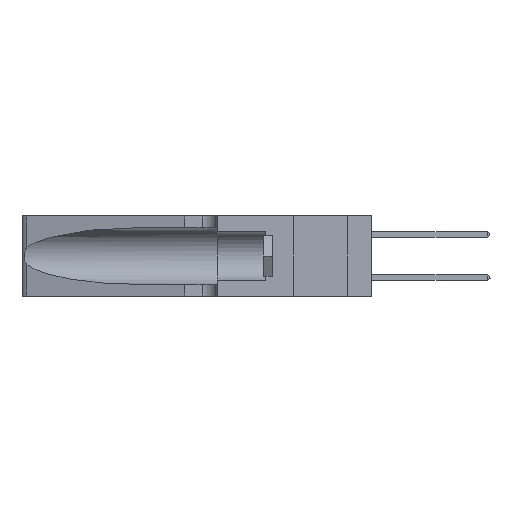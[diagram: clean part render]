
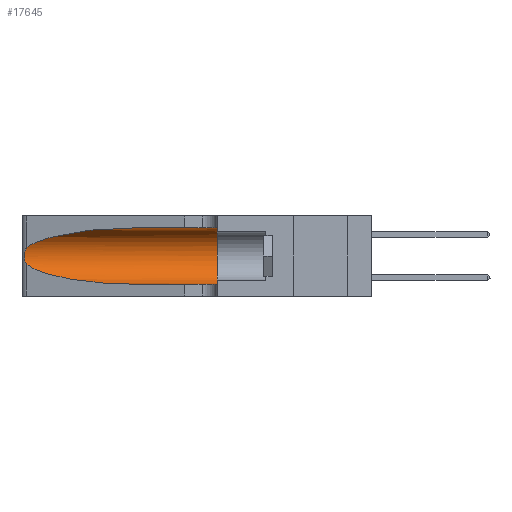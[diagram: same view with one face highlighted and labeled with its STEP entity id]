
A CAD part, left-side view. The second image highlights one B-rep face of the part: STEP entity #17645.
In plain terms, the highlighted cylindrical face has radius 3.308 mm (diameter 6.617 mm), a partial arc.
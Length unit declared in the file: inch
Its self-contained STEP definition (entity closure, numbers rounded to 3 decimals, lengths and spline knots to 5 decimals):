
#601 = CARTESIAN_POINT ( 'NONE',  ( 0.25789, 1.23486, 0.15765 ) ) ;
#664 = EDGE_CURVE ( 'NONE', #21509, #12738, #28038, .T. ) ;
#1256 = VECTOR ( 'NONE', #7456, 39.37008 ) ;
#2306 = CARTESIAN_POINT ( 'NONE',  ( 0.25487, 1.22718, 0.22369 ) ) ;
#3227 = CARTESIAN_POINT ( 'NONE',  ( 0.1305, 0.72297, 0.31525 ) ) ;
#3521 = CARTESIAN_POINT ( 'NONE',  ( 0.1305, 1.61858, 0.05475 ) ) ;
#4087 = FACE_OUTER_BOUND ( 'NONE', #15825, .T. ) ;
#4852 = CARTESIAN_POINT ( 'NONE',  ( 0.1305, 1.61858, 0.31525 ) ) ;
#5304 = AXIS2_PLACEMENT_3D ( 'NONE', #11814, #27728, #27369 ) ;
#5886 = ORIENTED_EDGE ( 'NONE', *, *, #25168, .T. ) ;
#6325 = DIRECTION ( 'NONE',  ( 0., -1., 0. ) ) ;
#6662 = CARTESIAN_POINT ( 'NONE',  ( 0.25487, 1.22718, 0.14631 ) ) ;
#6696 =( BOUNDED_CURVE ( )  B_SPLINE_CURVE ( 3, ( #14615, #17452, #19934, #24827 ),
 .UNSPECIFIED., .F., .F. ) 
 B_SPLINE_CURVE_WITH_KNOTS ( ( 4, 4 ),
 ( 1.5708, 2.84003 ),
 .UNSPECIFIED. ) 
 CURVE ( )  GEOMETRIC_REPRESENTATION_ITEM ( )  RATIONAL_B_SPLINE_CURVE ( ( 1., 0.87, 0.87, 1. ) ) 
 REPRESENTATION_ITEM ( '' )  );
#7092 = CARTESIAN_POINT ( 'NONE',  ( 0.1305, 0.72297, 0.05475 ) ) ;
#7456 = DIRECTION ( 'NONE',  ( 0., -1., 0. ) ) ;
#7496 = CARTESIAN_POINT ( 'NONE',  ( 0.26018, 1.23835, 0.19895 ) ) ;
#8985 = CARTESIAN_POINT ( 'NONE',  ( 0.25487, 1.22718, 0.14631 ) ) ;
#9748 = CARTESIAN_POINT ( 'NONE',  ( 0.25555, 1.22994, 0.2215 ) ) ;
#10372 = ORIENTED_EDGE ( 'NONE', *, *, #21077, .T. ) ;
#10446 = EDGE_CURVE ( 'NONE', #28811, #21509, #25939, .T. ) ;
#10840 = VERTEX_POINT ( 'NONE', #25632 ) ;
#11349 = CARTESIAN_POINT ( 'NONE',  ( 0.1305, 0.72297, 0.05475 ) ) ;
#11554 = LINE ( 'NONE', #3521, #21632 ) ;
#11681 = DIRECTION ( 'NONE',  ( 0., -1., 0. ) ) ;
#11778 = CIRCLE ( 'NONE', #5304, 0.13025 ) ;
#11814 = CARTESIAN_POINT ( 'NONE',  ( 0.1305, 0.35, 0.185 ) ) ;
#12738 = VERTEX_POINT ( 'NONE', #7092 ) ;
#14615 = CARTESIAN_POINT ( 'NONE',  ( 0.1305, 0.72297, 0.31525 ) ) ;
#14930 = CARTESIAN_POINT ( 'NONE',  ( 0.26017, 1.23833, 0.17102 ) ) ;
#14951 = ORIENTED_EDGE ( 'NONE', *, *, #29182, .F. ) ;
#15768 = CYLINDRICAL_SURFACE ( 'NONE', #17881, 0.13025 ) ;
#15825 = EDGE_LOOP ( 'NONE', ( #5886, #29830, #28706, #10372, #16165, #14951 ) ) ;
#16165 = ORIENTED_EDGE ( 'NONE', *, *, #17404, .F. ) ;
#16203 = VERTEX_POINT ( 'NONE', #17660 ) ;
#17404 = EDGE_CURVE ( 'NONE', #16203, #10840, #11778, .T. ) ;
#17430 = LINE ( 'NONE', #4852, #1256 ) ;
#17452 = CARTESIAN_POINT ( 'NONE',  ( 0.18966, 0.96281, 0.31525 ) ) ;
#17645 = ADVANCED_FACE ( 'NONE', ( #4087 ), #15768, .F. ) ;
#17660 = CARTESIAN_POINT ( 'NONE',  ( 0.1305, 0.35, 0.31525 ) ) ;
#17865 = CARTESIAN_POINT ( 'NONE',  ( 0.25787, 1.23484, 0.2124 ) ) ;
#17881 = AXIS2_PLACEMENT_3D ( 'NONE', #23623, #11681, #32170 ) ;
#17935 = CARTESIAN_POINT ( 'NONE',  ( 0.25856, 1.23593, 0.16098 ) ) ;
#19042 = CARTESIAN_POINT ( 'NONE',  ( 0.25487, 1.22718, 0.22369 ) ) ;
#19075 = VERTEX_POINT ( 'NONE', #3227 ) ;
#19934 = CARTESIAN_POINT ( 'NONE',  ( 0.2373, 1.15595, 0.28018 ) ) ;
#21077 = EDGE_CURVE ( 'NONE', #12738, #10840, #11554, .T. ) ;
#21247 = CARTESIAN_POINT ( 'NONE',  ( 0.25639, 1.23186, 0.15144 ) ) ;
#21509 = VERTEX_POINT ( 'NONE', #6662 ) ;
#21632 = VECTOR ( 'NONE', #6325, 39.37008 ) ;
#22580 = CARTESIAN_POINT ( 'NONE',  ( 0.26075, 1.23896, 0.19203 ) ) ;
#22929 = CARTESIAN_POINT ( 'NONE',  ( 0.25854, 1.2359, 0.20912 ) ) ;
#23623 = CARTESIAN_POINT ( 'NONE',  ( 0.1305, 1.61858, 0.185 ) ) ;
#24827 = CARTESIAN_POINT ( 'NONE',  ( 0.25487, 1.22718, 0.22369 ) ) ;
#25168 = EDGE_CURVE ( 'NONE', #19075, #28811, #6696, .T. ) ;
#25632 = CARTESIAN_POINT ( 'NONE',  ( 0.1305, 0.35, 0.05475 ) ) ;
#25939 = B_SPLINE_CURVE_WITH_KNOTS ( 'NONE', 3,
 ( #2306, #9748, #32837, #17865, #22929, #7496, #22580, #30347, #14930, #17935, #601, #21247, #29220, #29109 ),
 .UNSPECIFIED., .F., .F.,
 ( 4, 2, 2, 2, 2, 2, 4 ),
 ( 0., 0.00027, 0.00053, 0.00107, 0.0016, 0.00187, 0.00214 ),
 .UNSPECIFIED. ) ;
#27121 = CARTESIAN_POINT ( 'NONE',  ( 0.2373, 1.15595, 0.08982 ) ) ;
#27369 = DIRECTION ( 'NONE',  ( 0., 0., 1. ) ) ;
#27728 = DIRECTION ( 'NONE',  ( 0., 1., 0. ) ) ;
#28038 =( BOUNDED_CURVE ( )  B_SPLINE_CURVE ( 3, ( #8985, #27121, #29597, #11349 ),
 .UNSPECIFIED., .F., .F. ) 
 B_SPLINE_CURVE_WITH_KNOTS ( ( 4, 4 ),
 ( 3.44316, 4.71239 ),
 .UNSPECIFIED. ) 
 CURVE ( )  GEOMETRIC_REPRESENTATION_ITEM ( )  RATIONAL_B_SPLINE_CURVE ( ( 1., 0.87, 0.87, 1. ) ) 
 REPRESENTATION_ITEM ( '' )  );
#28706 = ORIENTED_EDGE ( 'NONE', *, *, #664, .T. ) ;
#28811 = VERTEX_POINT ( 'NONE', #19042 ) ;
#29109 = CARTESIAN_POINT ( 'NONE',  ( 0.25487, 1.22718, 0.14631 ) ) ;
#29182 = EDGE_CURVE ( 'NONE', #19075, #16203, #17430, .T. ) ;
#29220 = CARTESIAN_POINT ( 'NONE',  ( 0.25555, 1.22993, 0.14849 ) ) ;
#29597 = CARTESIAN_POINT ( 'NONE',  ( 0.18966, 0.96281, 0.05475 ) ) ;
#29830 = ORIENTED_EDGE ( 'NONE', *, *, #10446, .T. ) ;
#30347 = CARTESIAN_POINT ( 'NONE',  ( 0.26075, 1.23896, 0.178 ) ) ;
#32170 = DIRECTION ( 'NONE',  ( 0., 0., -1. ) ) ;
#32837 = CARTESIAN_POINT ( 'NONE',  ( 0.25639, 1.23184, 0.21858 ) ) ;
